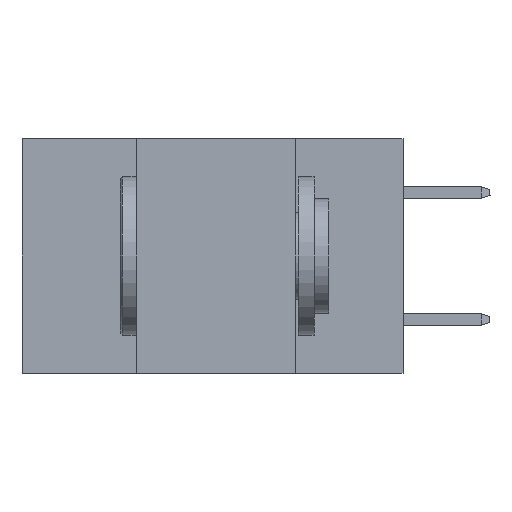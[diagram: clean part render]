
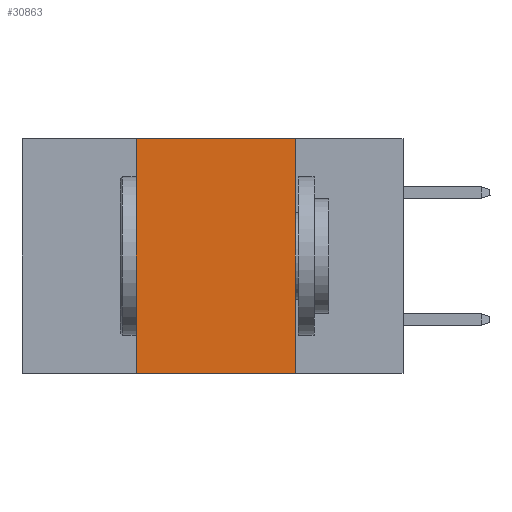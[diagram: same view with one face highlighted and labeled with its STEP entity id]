
A CAD part, left-side view. The second image highlights one B-rep face of the part: STEP entity #30863.
In plain terms, the highlighted planar face has unit normal (-1, 0, 0).
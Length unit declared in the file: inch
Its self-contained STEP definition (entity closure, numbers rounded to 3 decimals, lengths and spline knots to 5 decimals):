
#1262 = VECTOR ( 'NONE', #13619, 39.37008 ) ;
#1650 = ORIENTED_EDGE ( 'NONE', *, *, #42860, .T. ) ;
#1862 = PLANE ( 'NONE',  #25299 ) ;
#2758 = VERTEX_POINT ( 'NONE', #32258 ) ;
#3464 = ORIENTED_EDGE ( 'NONE', *, *, #31694, .F. ) ;
#5989 = VECTOR ( 'NONE', #24433, 39.37008 ) ;
#6119 = DIRECTION ( 'NONE',  ( 0., 0., -1. ) ) ;
#6473 = CARTESIAN_POINT ( 'NONE',  ( 0., 0.6, 0. ) ) ;
#7164 = CARTESIAN_POINT ( 'NONE',  ( 0., 0.42, 0. ) ) ;
#8462 = VERTEX_POINT ( 'NONE', #39529 ) ;
#9690 = ORIENTED_EDGE ( 'NONE', *, *, #35508, .F. ) ;
#10888 = EDGE_CURVE ( 'NONE', #41918, #27759, #17411, .T. ) ;
#11247 = ORIENTED_EDGE ( 'NONE', *, *, #10888, .F. ) ;
#13619 = DIRECTION ( 'NONE',  ( 0., -1., 0. ) ) ;
#15953 = FACE_OUTER_BOUND ( 'NONE', #27224, .T. ) ;
#17411 = LINE ( 'NONE', #6473, #1262 ) ;
#17689 = LINE ( 'NONE', #35148, #26903 ) ;
#20156 = LINE ( 'NONE', #44112, #27602 ) ;
#20258 = CARTESIAN_POINT ( 'NONE',  ( 0., 0.17, 0. ) ) ;
#23154 = DIRECTION ( 'NONE',  ( 1., 0., 0. ) ) ;
#24433 = DIRECTION ( 'NONE',  ( 0., 0., 1. ) ) ;
#24447 = DIRECTION ( 'NONE',  ( 0., -1., 0. ) ) ;
#25299 = AXIS2_PLACEMENT_3D ( 'NONE', #39279, #23154, #6119 ) ;
#26903 = VECTOR ( 'NONE', #24447, 39.37008 ) ;
#27224 = EDGE_LOOP ( 'NONE', ( #9690, #11247, #3464, #1650 ) ) ;
#27602 = VECTOR ( 'NONE', #29791, 39.37008 ) ;
#27759 = VERTEX_POINT ( 'NONE', #20258 ) ;
#29791 = DIRECTION ( 'NONE',  ( 0., 0., -1. ) ) ;
#30863 = ADVANCED_FACE ( 'NONE', ( #15953 ), #1862, .F. ) ;
#31354 = LINE ( 'NONE', #7164, #5989 ) ;
#31694 = EDGE_CURVE ( 'NONE', #8462, #41918, #31354, .T. ) ;
#32258 = CARTESIAN_POINT ( 'NONE',  ( 0., 0.17, -0.37 ) ) ;
#34802 = CARTESIAN_POINT ( 'NONE',  ( 0., 0.42, 0. ) ) ;
#35148 = CARTESIAN_POINT ( 'NONE',  ( 0., 0.6, -0.37 ) ) ;
#35508 = EDGE_CURVE ( 'NONE', #27759, #2758, #20156, .T. ) ;
#39279 = CARTESIAN_POINT ( 'NONE',  ( 0., 0.6, 0. ) ) ;
#39529 = CARTESIAN_POINT ( 'NONE',  ( 0., 0.42, -0.37 ) ) ;
#41918 = VERTEX_POINT ( 'NONE', #34802 ) ;
#42860 = EDGE_CURVE ( 'NONE', #8462, #2758, #17689, .T. ) ;
#44112 = CARTESIAN_POINT ( 'NONE',  ( 0., 0.17, 0. ) ) ;
